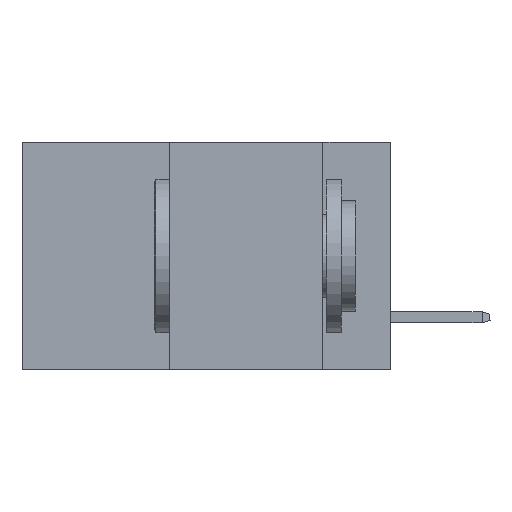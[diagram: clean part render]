
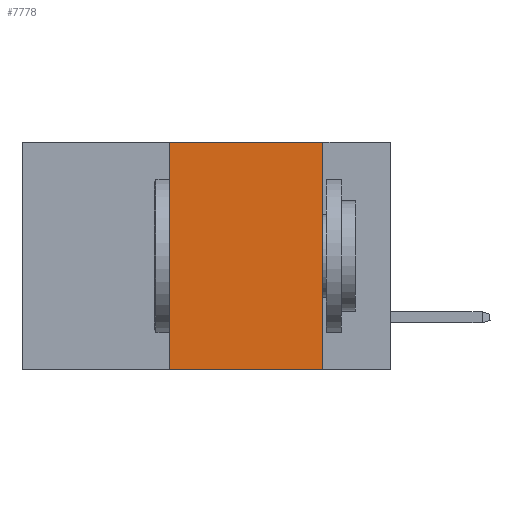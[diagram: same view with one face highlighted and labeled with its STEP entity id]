
A CAD part, left-side view. The second image highlights one B-rep face of the part: STEP entity #7778.
In plain terms, the highlighted planar face has unit normal (-1, 0, 0).
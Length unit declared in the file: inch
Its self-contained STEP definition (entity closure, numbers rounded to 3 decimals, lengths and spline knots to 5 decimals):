
#930 = VERTEX_POINT ( 'NONE', #19139 ) ;
#1642 = CARTESIAN_POINT ( 'NONE',  ( 0., 0.6, 0. ) ) ;
#2306 = CARTESIAN_POINT ( 'NONE',  ( 0., 0.11, 0. ) ) ;
#3629 = DIRECTION ( 'NONE',  ( 0., 0., -1. ) ) ;
#3799 = EDGE_CURVE ( 'NONE', #14316, #930, #6582, .T. ) ;
#3862 = DIRECTION ( 'NONE',  ( 0., 0., 1. ) ) ;
#4148 = FACE_OUTER_BOUND ( 'NONE', #16491, .T. ) ;
#4164 = CARTESIAN_POINT ( 'NONE',  ( 0., 0.6, -0.37 ) ) ;
#4266 = ORIENTED_EDGE ( 'NONE', *, *, #5696, .F. ) ;
#5323 = EDGE_CURVE ( 'NONE', #17583, #930, #18408, .T. ) ;
#5329 = VECTOR ( 'NONE', #20013, 39.37008 ) ;
#5696 = EDGE_CURVE ( 'NONE', #17583, #16950, #17894, .T. ) ;
#6097 = VECTOR ( 'NONE', #3629, 39.37008 ) ;
#6176 = PLANE ( 'NONE',  #10521 ) ;
#6582 = LINE ( 'NONE', #2306, #6097 ) ;
#6830 = ORIENTED_EDGE ( 'NONE', *, *, #3799, .F. ) ;
#7174 = CARTESIAN_POINT ( 'NONE',  ( 0., 0.36, 0. ) ) ;
#7778 = ADVANCED_FACE ( 'NONE', ( #4148 ), #6176, .F. ) ;
#10521 = AXIS2_PLACEMENT_3D ( 'NONE', #17052, #10870, #15594 ) ;
#10870 = DIRECTION ( 'NONE',  ( 1., 0., 0. ) ) ;
#12881 = EDGE_CURVE ( 'NONE', #16950, #14316, #19610, .T. ) ;
#14316 = VERTEX_POINT ( 'NONE', #15032 ) ;
#15032 = CARTESIAN_POINT ( 'NONE',  ( 0., 0.11, 0. ) ) ;
#15258 = VECTOR ( 'NONE', #3862, 39.37008 ) ;
#15594 = DIRECTION ( 'NONE',  ( 0., 0., -1. ) ) ;
#15693 = DIRECTION ( 'NONE',  ( 0., -1., 0. ) ) ;
#16491 = EDGE_LOOP ( 'NONE', ( #6830, #18866, #4266, #19975 ) ) ;
#16950 = VERTEX_POINT ( 'NONE', #7174 ) ;
#17052 = CARTESIAN_POINT ( 'NONE',  ( 0., 0.6, 0. ) ) ;
#17583 = VERTEX_POINT ( 'NONE', #18745 ) ;
#17894 = LINE ( 'NONE', #19274, #15258 ) ;
#18408 = LINE ( 'NONE', #4164, #5329 ) ;
#18745 = CARTESIAN_POINT ( 'NONE',  ( 0., 0.36, -0.37 ) ) ;
#18866 = ORIENTED_EDGE ( 'NONE', *, *, #12881, .F. ) ;
#19139 = CARTESIAN_POINT ( 'NONE',  ( 0., 0.11, -0.37 ) ) ;
#19274 = CARTESIAN_POINT ( 'NONE',  ( 0., 0.36, 0. ) ) ;
#19610 = LINE ( 'NONE', #1642, #20107 ) ;
#19975 = ORIENTED_EDGE ( 'NONE', *, *, #5323, .T. ) ;
#20013 = DIRECTION ( 'NONE',  ( 0., -1., 0. ) ) ;
#20107 = VECTOR ( 'NONE', #15693, 39.37008 ) ;
